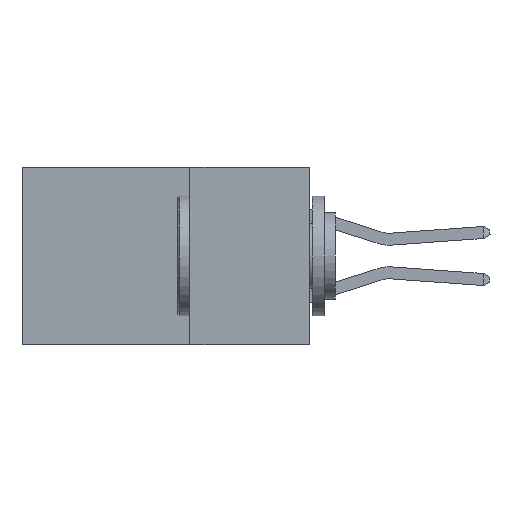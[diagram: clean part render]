
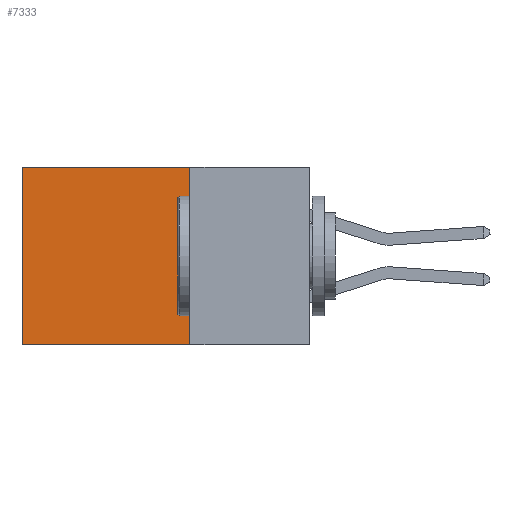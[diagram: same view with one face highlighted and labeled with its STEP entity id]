
A CAD part, left-side view. The second image highlights one B-rep face of the part: STEP entity #7333.
In plain terms, the highlighted planar face has unit normal (-1, 0, 0).
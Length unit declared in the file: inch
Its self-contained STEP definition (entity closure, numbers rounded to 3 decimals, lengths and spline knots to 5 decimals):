
#282 = VECTOR ( 'NONE', #2396, 39.37008 ) ;
#546 = EDGE_CURVE ( 'NONE', #2970, #650, #4680, .T. ) ;
#650 = VERTEX_POINT ( 'NONE', #5679 ) ;
#1139 = CARTESIAN_POINT ( 'NONE',  ( 0.298, 0.25, -0.37 ) ) ;
#2083 = CARTESIAN_POINT ( 'NONE',  ( 0.298, 0.25, 0. ) ) ;
#2088 = VECTOR ( 'NONE', #2683, 39.37008 ) ;
#2394 = CARTESIAN_POINT ( 'NONE',  ( 0.298, 0.25, -0.37 ) ) ;
#2396 = DIRECTION ( 'NONE',  ( 0., 0., -1. ) ) ;
#2660 = EDGE_CURVE ( 'NONE', #8035, #2970, #8257, .T. ) ;
#2683 = DIRECTION ( 'NONE',  ( 0., 1., 0. ) ) ;
#2772 = EDGE_LOOP ( 'NONE', ( #7965, #4193, #3566, #3873 ) ) ;
#2913 = CARTESIAN_POINT ( 'NONE',  ( 0.298, 0.25, 0. ) ) ;
#2970 = VERTEX_POINT ( 'NONE', #3487 ) ;
#3417 = CARTESIAN_POINT ( 'NONE',  ( 0.298, 0.25, 0. ) ) ;
#3487 = CARTESIAN_POINT ( 'NONE',  ( 0.298, 0.6, 0. ) ) ;
#3566 = ORIENTED_EDGE ( 'NONE', *, *, #5446, .F. ) ;
#3829 = VECTOR ( 'NONE', #4273, 39.37008 ) ;
#3873 = ORIENTED_EDGE ( 'NONE', *, *, #2660, .T. ) ;
#3902 = CARTESIAN_POINT ( 'NONE',  ( 0.298, 0.25, 0. ) ) ;
#4193 = ORIENTED_EDGE ( 'NONE', *, *, #7508, .F. ) ;
#4273 = DIRECTION ( 'NONE',  ( 0., 1., 0. ) ) ;
#4469 = LINE ( 'NONE', #3902, #5916 ) ;
#4670 = DIRECTION ( 'NONE',  ( 0., 0., -1. ) ) ;
#4680 = LINE ( 'NONE', #8490, #282 ) ;
#5446 = EDGE_CURVE ( 'NONE', #8035, #6369, #4469, .T. ) ;
#5472 = DIRECTION ( 'NONE',  ( 0., 0., -1. ) ) ;
#5679 = CARTESIAN_POINT ( 'NONE',  ( 0.298, 0.6, -0.37 ) ) ;
#5916 = VECTOR ( 'NONE', #4670, 39.37008 ) ;
#6369 = VERTEX_POINT ( 'NONE', #2394 ) ;
#6730 = FACE_OUTER_BOUND ( 'NONE', #2772, .T. ) ;
#7333 = ADVANCED_FACE ( 'NONE', ( #6730 ), #7604, .F. ) ;
#7508 = EDGE_CURVE ( 'NONE', #6369, #650, #7818, .T. ) ;
#7604 = PLANE ( 'NONE',  #8574 ) ;
#7818 = LINE ( 'NONE', #1139, #3829 ) ;
#7965 = ORIENTED_EDGE ( 'NONE', *, *, #546, .T. ) ;
#8035 = VERTEX_POINT ( 'NONE', #2083 ) ;
#8257 = LINE ( 'NONE', #3417, #2088 ) ;
#8427 = DIRECTION ( 'NONE',  ( 1., 0., 0. ) ) ;
#8490 = CARTESIAN_POINT ( 'NONE',  ( 0.298, 0.6, 0. ) ) ;
#8574 = AXIS2_PLACEMENT_3D ( 'NONE', #2913, #8427, #5472 ) ;
